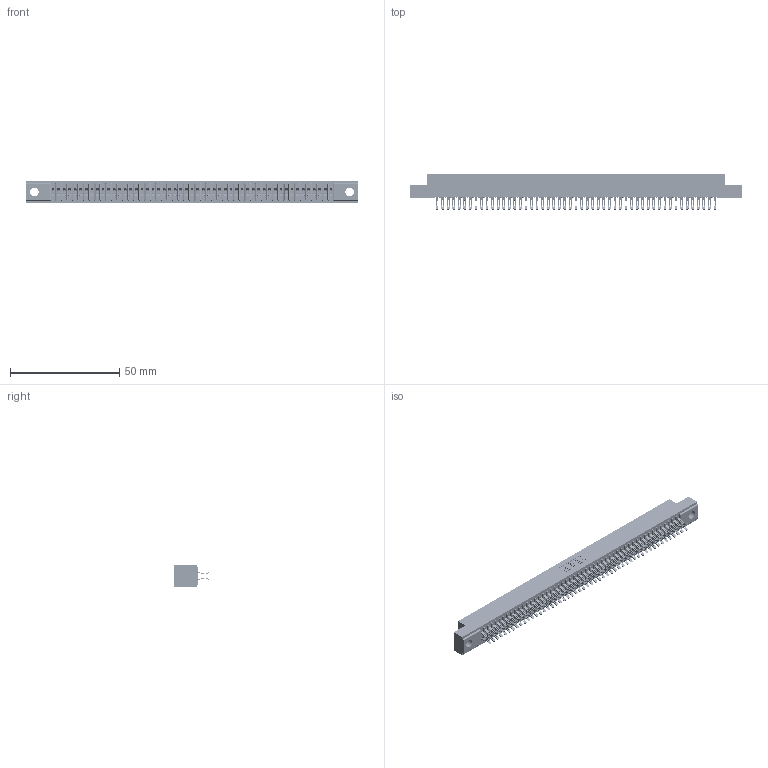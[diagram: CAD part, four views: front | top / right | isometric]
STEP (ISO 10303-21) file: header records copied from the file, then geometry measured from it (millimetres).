
FILE_DESCRIPTION (( 'STEP AP203' ), '1' );
FILE_NAME ('391-102-555-204.STEP', '2018-08-09T20:01:10', ( '' ), ( '' ), 'SwSTEP 2.0', 'SolidWorks 2016', '' );
FILE_SCHEMA (( 'CONFIG_CONTROL_DESIGN' ));
Length unit declared in the file: inch
Products named in the file (3): 341 Part_.156 (3.96) Dia Mounting Holes; 341-292-001_341-292-155; 391-102-555-204
Assembly tree (103 placements, depth 2):
  391-102-555-204
    341 Part_.156 (3.96) Dia Mounting Holes
    341-292-001_341-292-155  x102
Bounding box: 151.76 x 16.31 x 10.16 mm (x, y, z)
Volume: 11238.7 mm3; surface area: 20953.1 mm2
Topology: 103 solids, 103 shells, 8086 faces, 24169 edges, 15734 vertices
Faces by surface type: plane 4366, cylinder 3516, sphere 104, torus 100
Entity records: 61410 total; most frequent: CARTESIAN_POINT 10229, ORIENTED_EDGE 10154, DIRECTION 9903, EDGE_CURVE 5077, LINE 4103, VECTOR 4103, VERTEX_POINT 3210, AXIS2_PLACEMENT_3D 2900
